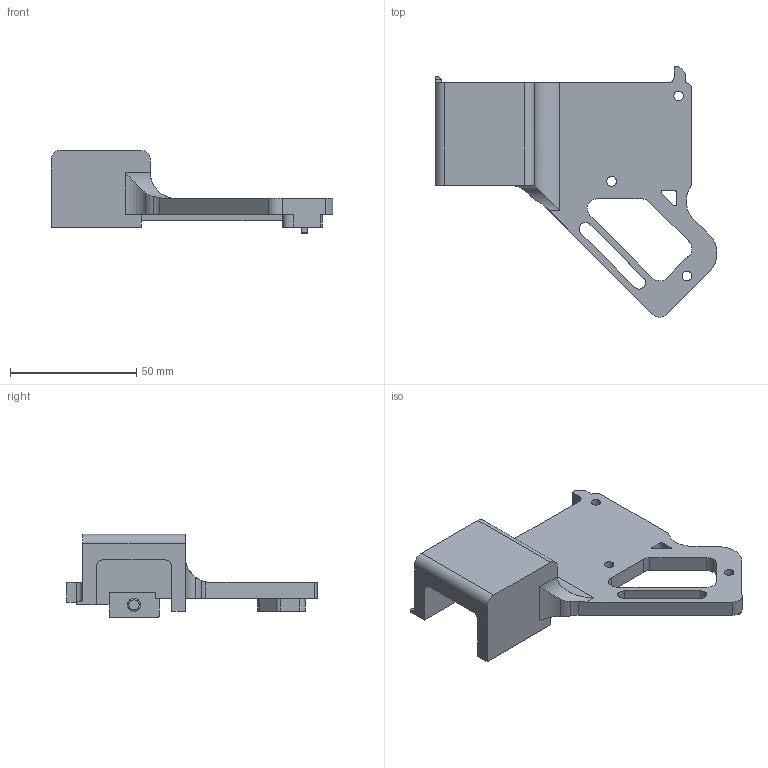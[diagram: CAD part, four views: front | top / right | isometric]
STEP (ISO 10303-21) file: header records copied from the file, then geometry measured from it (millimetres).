
FILE_DESCRIPTION (( 'STEP AP214' ), '1' );
FILE_NAME ('frame_r.STEP', '2014-01-22T21:33:40', ( '' ), ( '' ), 'SwSTEP 2.0', 'SolidWorks 2013', '' );
FILE_SCHEMA (( 'AUTOMOTIVE_DESIGN' ));
Length unit declared in the file: inch
Products named in the file (1): frame_r
Bounding box: 111.75 x 99.3 x 33.02 mm (x, y, z)
Volume: 50138.6 mm3; surface area: 20806.3 mm2
Topology: 1 solids, 1 shells, 104 faces, 294 edges, 193 vertices
Faces by surface type: plane 56, cylinder 46, torus 2
Entity records: 3448 total; most frequent: CARTESIAN_POINT 613, DIRECTION 589, ORIENTED_EDGE 588, EDGE_CURVE 294, VECTOR 199, LINE 199, AXIS2_PLACEMENT_3D 195, VERTEX_POINT 193
